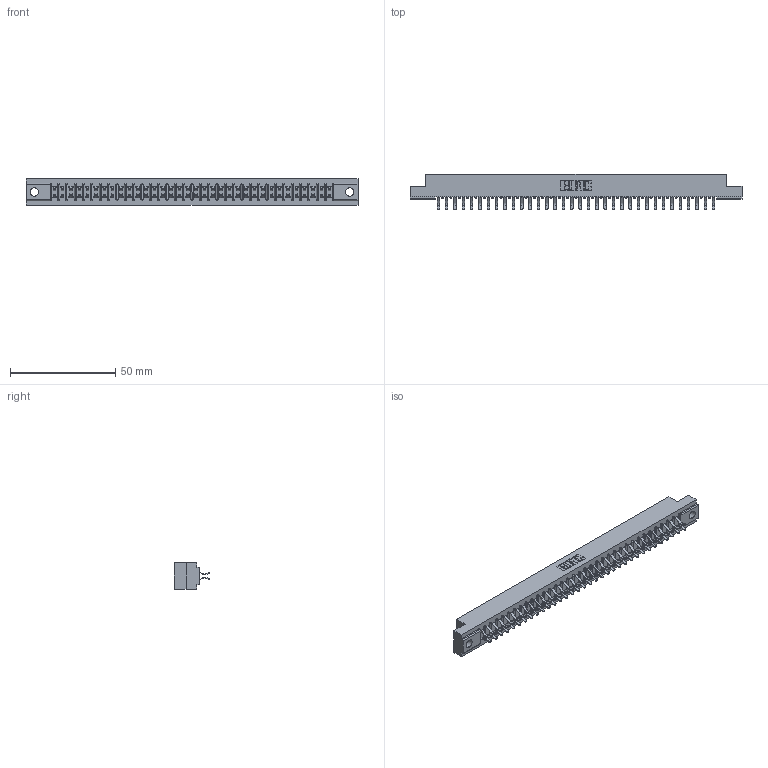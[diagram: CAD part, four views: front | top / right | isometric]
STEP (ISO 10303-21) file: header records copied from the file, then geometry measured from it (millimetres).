
FILE_DESCRIPTION (( 'STEP AP203' ), '1' );
FILE_NAME ('357-068-556-204.STEP', '2019-09-19T09:44:45', ( '' ), ( '' ), 'SwSTEP 2.0', 'SolidWorks 2016', '' );
FILE_SCHEMA (( 'CONFIG_CONTROL_DESIGN' ));
Length unit declared in the file: inch
Products named in the file (3): 307 Part_.156 Dia Mounting Holes; 307-290-001_556; 357-068-556-204
Assembly tree (69 placements, depth 2):
  357-068-556-204
    307 Part_.156 Dia Mounting Holes
    307-290-001_556  x68
Bounding box: 157.73 x 16.97 x 12.7 mm (x, y, z)
Volume: 16598.2 mm3; surface area: 19801.7 mm2
Topology: 69 solids, 69 shells, 3567 faces, 10015 edges, 6490 vertices
Faces by surface type: plane 2328, cylinder 1169, sphere 70
Entity records: 31744 total; most frequent: CARTESIAN_POINT 5200, ORIENTED_EDGE 5150, DIRECTION 5089, EDGE_CURVE 2575, VECTOR 1979, LINE 1979, VERTEX_POINT 1666, AXIS2_PLACEMENT_3D 1555
